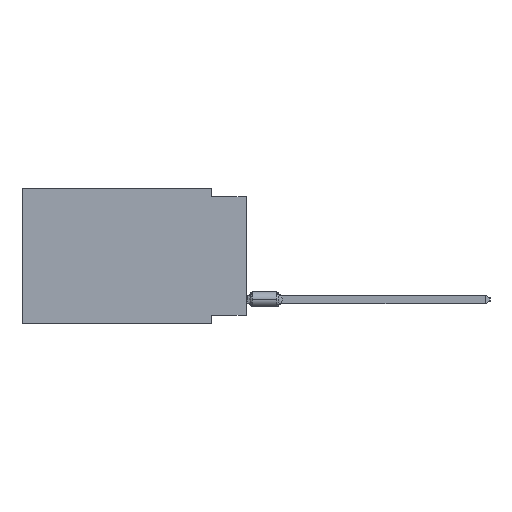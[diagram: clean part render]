
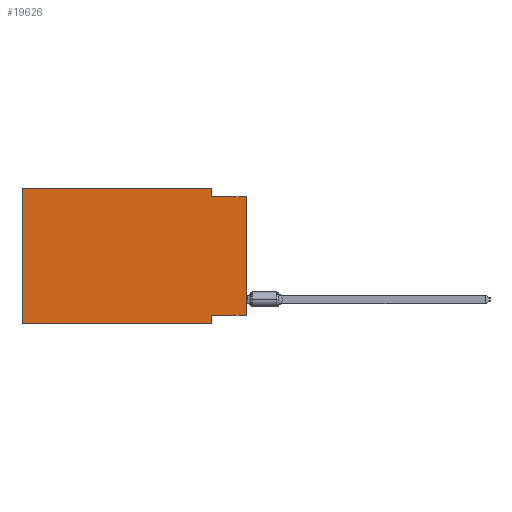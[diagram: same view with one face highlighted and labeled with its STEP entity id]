
A CAD part, left-side view. The second image highlights one B-rep face of the part: STEP entity #19626.
In plain terms, the highlighted planar face has unit normal (-1, 0, 0).
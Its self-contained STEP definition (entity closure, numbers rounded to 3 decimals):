
#1327 = VERTEX_POINT ( 'NONE', #67251 ) ;
#2854 = LINE ( 'NONE', #46198, #16557 ) ;
#2858 = CARTESIAN_POINT ( 'NONE',  ( 0., 0., 0. ) ) ;
#3174 = ORIENTED_EDGE ( 'NONE', *, *, #52028, .F. ) ;
#3987 = ORIENTED_EDGE ( 'NONE', *, *, #64638, .F. ) ;
#5600 = VECTOR ( 'NONE', #37111, 1000. ) ;
#5997 = EDGE_CURVE ( 'NONE', #57873, #41930, #29481, .T. ) ;
#7550 = DIRECTION ( 'NONE',  ( 0., -1., 0. ) ) ;
#7987 = CARTESIAN_POINT ( 'NONE',  ( 0., 16.383, 0. ) ) ;
#8550 = ORIENTED_EDGE ( 'NONE', *, *, #55539, .F. ) ;
#10119 = CARTESIAN_POINT ( 'NONE',  ( 0., 2.54, -9.906 ) ) ;
#10960 = VERTEX_POINT ( 'NONE', #42801 ) ;
#12243 = CARTESIAN_POINT ( 'NONE',  ( 0., 0., -9.271 ) ) ;
#16557 = VECTOR ( 'NONE', #46544, 1000. ) ;
#16895 = CARTESIAN_POINT ( 'NONE',  ( 0., 2.54, 0. ) ) ;
#17111 = VECTOR ( 'NONE', #50863, 1000. ) ;
#18821 = DIRECTION ( 'NONE',  ( 0., 0., 1. ) ) ;
#18965 = CARTESIAN_POINT ( 'NONE',  ( 0., 16.383, 0. ) ) ;
#19626 = ADVANCED_FACE ( 'NONE', ( #33406 ), #54377, .F. ) ;
#21537 = DIRECTION ( 'NONE',  ( 0., 0., -1. ) ) ;
#21550 = VERTEX_POINT ( 'NONE', #67192 ) ;
#21655 = VECTOR ( 'NONE', #21537, 1000. ) ;
#22533 = CARTESIAN_POINT ( 'NONE',  ( 0., 0., -0.635 ) ) ;
#28414 = AXIS2_PLACEMENT_3D ( 'NONE', #33040, #38727, #43725 ) ;
#29481 = LINE ( 'NONE', #2858, #60606 ) ;
#29817 = EDGE_CURVE ( 'NONE', #21550, #1327, #51240, .T. ) ;
#31092 = EDGE_CURVE ( 'NONE', #31564, #37769, #46246, .T. ) ;
#31564 = VERTEX_POINT ( 'NONE', #18965 ) ;
#32219 = LINE ( 'NONE', #53913, #21655 ) ;
#32538 = ORIENTED_EDGE ( 'NONE', *, *, #31092, .F. ) ;
#32655 = ORIENTED_EDGE ( 'NONE', *, *, #52254, .F. ) ;
#33040 = CARTESIAN_POINT ( 'NONE',  ( 0., 16.383, 0. ) ) ;
#33406 = FACE_OUTER_BOUND ( 'NONE', #54686, .T. ) ;
#34531 = CARTESIAN_POINT ( 'NONE',  ( 0., 16.383, -9.906 ) ) ;
#34539 = CARTESIAN_POINT ( 'NONE',  ( 0., 16.383, 0. ) ) ;
#37111 = DIRECTION ( 'NONE',  ( 0., 0., -1. ) ) ;
#37769 = VERTEX_POINT ( 'NONE', #16895 ) ;
#38727 = DIRECTION ( 'NONE',  ( 1., 0., 0. ) ) ;
#39858 = DIRECTION ( 'NONE',  ( 0., -1., 0. ) ) ;
#39950 = DIRECTION ( 'NONE',  ( 0., 0., 1. ) ) ;
#40821 = VECTOR ( 'NONE', #7550, 1000. ) ;
#40831 = EDGE_CURVE ( 'NONE', #21550, #31564, #67012, .T. ) ;
#41930 = VERTEX_POINT ( 'NONE', #22533 ) ;
#42801 = CARTESIAN_POINT ( 'NONE',  ( 0., 2.54, -0.635 ) ) ;
#43399 = ORIENTED_EDGE ( 'NONE', *, *, #5997, .T. ) ;
#43725 = DIRECTION ( 'NONE',  ( 0., 0., -1. ) ) ;
#46198 = CARTESIAN_POINT ( 'NONE',  ( 0., 0., -9.271 ) ) ;
#46246 = LINE ( 'NONE', #34539, #40821 ) ;
#46544 = DIRECTION ( 'NONE',  ( 0., 1., 0. ) ) ;
#50165 = LINE ( 'NONE', #50527, #17111 ) ;
#50527 = CARTESIAN_POINT ( 'NONE',  ( 0., 0., -0.635 ) ) ;
#50863 = DIRECTION ( 'NONE',  ( 0., -1., 0. ) ) ;
#51240 = LINE ( 'NONE', #34531, #55432 ) ;
#52028 = EDGE_CURVE ( 'NONE', #10960, #41930, #50165, .T. ) ;
#52254 = EDGE_CURVE ( 'NONE', #37769, #10960, #32219, .T. ) ;
#53913 = CARTESIAN_POINT ( 'NONE',  ( 0., 2.54, 0. ) ) ;
#54377 = PLANE ( 'NONE',  #28414 ) ;
#54686 = EDGE_LOOP ( 'NONE', ( #43399, #3174, #32655, #32538, #60170, #70106, #3987, #8550 ) ) ;
#55432 = VECTOR ( 'NONE', #39858, 1000. ) ;
#55539 = EDGE_CURVE ( 'NONE', #57873, #56386, #2854, .T. ) ;
#56386 = VERTEX_POINT ( 'NONE', #58469 ) ;
#57873 = VERTEX_POINT ( 'NONE', #12243 ) ;
#58469 = CARTESIAN_POINT ( 'NONE',  ( 0., 2.54, -9.271 ) ) ;
#59329 = VECTOR ( 'NONE', #39950, 1000. ) ;
#59838 = LINE ( 'NONE', #10119, #5600 ) ;
#60170 = ORIENTED_EDGE ( 'NONE', *, *, #40831, .F. ) ;
#60606 = VECTOR ( 'NONE', #18821, 1000. ) ;
#64638 = EDGE_CURVE ( 'NONE', #56386, #1327, #59838, .T. ) ;
#67012 = LINE ( 'NONE', #7987, #59329 ) ;
#67192 = CARTESIAN_POINT ( 'NONE',  ( 0., 16.383, -9.906 ) ) ;
#67251 = CARTESIAN_POINT ( 'NONE',  ( 0., 2.54, -9.906 ) ) ;
#70106 = ORIENTED_EDGE ( 'NONE', *, *, #29817, .T. ) ;
